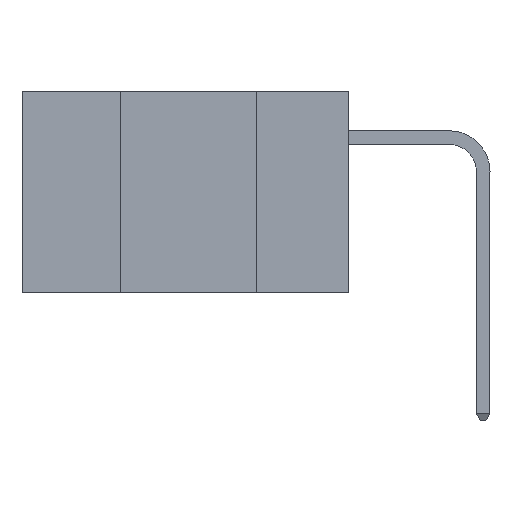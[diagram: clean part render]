
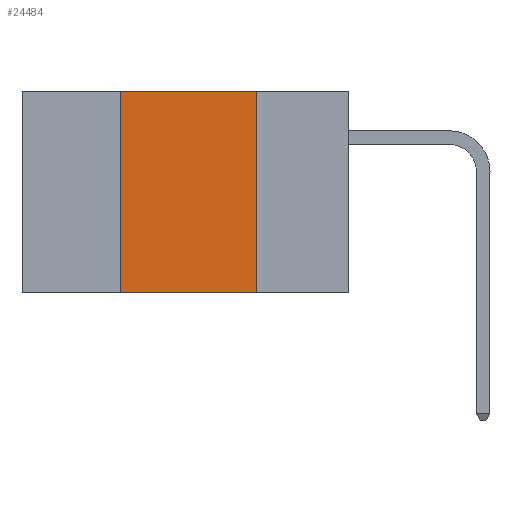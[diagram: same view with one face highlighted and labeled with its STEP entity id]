
A CAD part, left-side view. The second image highlights one B-rep face of the part: STEP entity #24484.
In plain terms, the highlighted planar face has unit normal (-1, 0, 0).
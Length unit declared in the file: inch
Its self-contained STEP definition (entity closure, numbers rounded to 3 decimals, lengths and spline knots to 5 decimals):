
#164 = LINE ( 'NONE', #12319, #14931 ) ;
#1183 = CARTESIAN_POINT ( 'NONE',  ( 0., 0.17, 0. ) ) ;
#1326 = CARTESIAN_POINT ( 'NONE',  ( 0., 0.42, -0.37 ) ) ;
#2710 = ORIENTED_EDGE ( 'NONE', *, *, #19910, .F. ) ;
#3209 = CARTESIAN_POINT ( 'NONE',  ( 0., 0.42, 0. ) ) ;
#3441 = VECTOR ( 'NONE', #9821, 39.37008 ) ;
#3979 = EDGE_CURVE ( 'NONE', #14596, #18231, #14213, .T. ) ;
#4849 = VERTEX_POINT ( 'NONE', #1326 ) ;
#5205 = EDGE_CURVE ( 'NONE', #4849, #18231, #9865, .T. ) ;
#5546 = DIRECTION ( 'NONE',  ( 0., -1., 0. ) ) ;
#5858 = EDGE_LOOP ( 'NONE', ( #11283, #2710, #14713, #14449 ) ) ;
#6157 = AXIS2_PLACEMENT_3D ( 'NONE', #21610, #11990, #23472 ) ;
#7511 = VERTEX_POINT ( 'NONE', #3209 ) ;
#8992 = VECTOR ( 'NONE', #5546, 39.37008 ) ;
#9821 = DIRECTION ( 'NONE',  ( 0., 0., 1. ) ) ;
#9865 = LINE ( 'NONE', #24713, #8992 ) ;
#11283 = ORIENTED_EDGE ( 'NONE', *, *, #3979, .F. ) ;
#11750 = PLANE ( 'NONE',  #6157 ) ;
#11779 = VECTOR ( 'NONE', #19242, 39.37008 ) ;
#11990 = DIRECTION ( 'NONE',  ( 1., 0., 0. ) ) ;
#12125 = FACE_OUTER_BOUND ( 'NONE', #5858, .T. ) ;
#12319 = CARTESIAN_POINT ( 'NONE',  ( 0., 0.6, 0. ) ) ;
#13946 = CARTESIAN_POINT ( 'NONE',  ( 0., 0.42, 0. ) ) ;
#14213 = LINE ( 'NONE', #17097, #11779 ) ;
#14449 = ORIENTED_EDGE ( 'NONE', *, *, #5205, .T. ) ;
#14596 = VERTEX_POINT ( 'NONE', #1183 ) ;
#14713 = ORIENTED_EDGE ( 'NONE', *, *, #24512, .F. ) ;
#14931 = VECTOR ( 'NONE', #22202, 39.37008 ) ;
#17097 = CARTESIAN_POINT ( 'NONE',  ( 0., 0.17, 0. ) ) ;
#18231 = VERTEX_POINT ( 'NONE', #24521 ) ;
#19242 = DIRECTION ( 'NONE',  ( 0., 0., -1. ) ) ;
#19910 = EDGE_CURVE ( 'NONE', #7511, #14596, #164, .T. ) ;
#21610 = CARTESIAN_POINT ( 'NONE',  ( 0., 0.6, 0. ) ) ;
#21870 = LINE ( 'NONE', #13946, #3441 ) ;
#22202 = DIRECTION ( 'NONE',  ( 0., -1., 0. ) ) ;
#23472 = DIRECTION ( 'NONE',  ( 0., 0., -1. ) ) ;
#24484 = ADVANCED_FACE ( 'NONE', ( #12125 ), #11750, .F. ) ;
#24512 = EDGE_CURVE ( 'NONE', #4849, #7511, #21870, .T. ) ;
#24521 = CARTESIAN_POINT ( 'NONE',  ( 0., 0.17, -0.37 ) ) ;
#24713 = CARTESIAN_POINT ( 'NONE',  ( 0., 0.6, -0.37 ) ) ;
